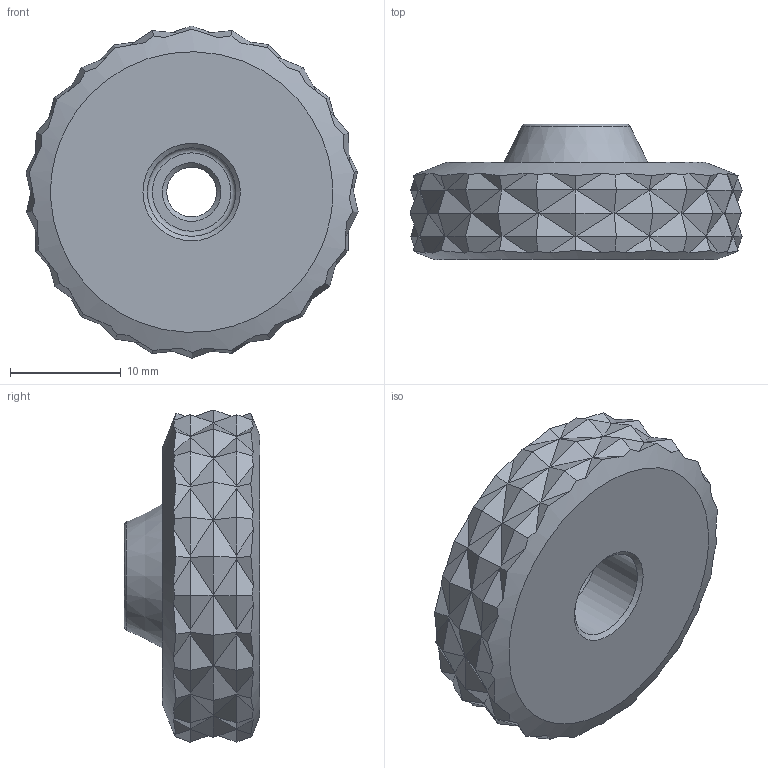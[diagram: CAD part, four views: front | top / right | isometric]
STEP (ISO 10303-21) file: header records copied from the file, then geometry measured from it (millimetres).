
FILE_DESCRIPTION (( 'STEP AP203' ), '1' );
FILE_NAME ('MOD9_G36_stock_knob.STEP', '2020-07-07T01:46:55', ( '' ), ( '' ), 'SwSTEP 2.0', 'SolidWorks 2016', '' );
FILE_SCHEMA (( 'CONFIG_CONTROL_DESIGN' ));
Length unit declared in the file: millimetre
Products named in the file (1): MOD9_G36_stock_knob
Bounding box: 30 x 12.23 x 30 mm (x, y, z)
Volume: 5529.3 mm3; surface area: 2301.5 mm2
Topology: 1 solids, 1 shells, 260 faces, 673 edges, 417 vertices
Faces by surface type: plane 251, cone 3, torus 2, cylinder 2, bspline 2
Full cylindrical faces by diameter (mm): 4.5 x1, 8 x1
Entity records: 7599 total; most frequent: CARTESIAN_POINT 1602, ORIENTED_EDGE 1324, DIRECTION 1082, EDGE_CURVE 662, LINE 544, VECTOR 544, VERTEX_POINT 415, EDGE_LOOP 273
